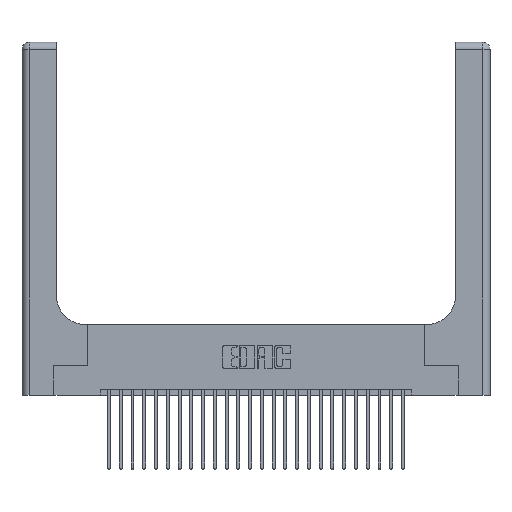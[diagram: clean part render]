
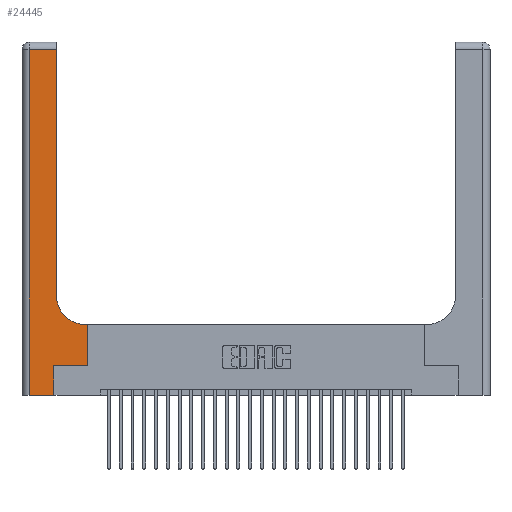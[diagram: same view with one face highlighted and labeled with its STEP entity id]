
A CAD part, top view. The second image highlights one B-rep face of the part: STEP entity #24445.
In plain terms, the highlighted planar face has unit normal (0, 0, 1).
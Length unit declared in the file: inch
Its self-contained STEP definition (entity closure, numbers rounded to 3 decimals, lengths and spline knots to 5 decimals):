
#80 = CARTESIAN_POINT ( 'NONE',  ( 0.06, 2.94, 0.37 ) ) ;
#193 = EDGE_CURVE ( 'NONE', #15924, #9389, #17839, .T. ) ;
#535 = CARTESIAN_POINT ( 'NONE',  ( 0.2915, 3., 0.37 ) ) ;
#788 = DIRECTION ( 'NONE',  ( 0., 1., 0. ) ) ;
#855 = EDGE_CURVE ( 'NONE', #9389, #20515, #4159, .T. ) ;
#867 = CARTESIAN_POINT ( 'NONE',  ( 0., 3., 0.37 ) ) ;
#1269 = VECTOR ( 'NONE', #12294, 39.37008 ) ;
#1270 = ORIENTED_EDGE ( 'NONE', *, *, #2714, .T. ) ;
#1662 = DIRECTION ( 'NONE',  ( 0., 1., 0. ) ) ;
#1924 = CARTESIAN_POINT ( 'NONE',  ( 0.5415, 0.85, 0.37 ) ) ;
#2631 = ORIENTED_EDGE ( 'NONE', *, *, #27684, .T. ) ;
#2714 = EDGE_CURVE ( 'NONE', #18409, #4987, #21042, .T. ) ;
#2763 = VECTOR ( 'NONE', #6389, 39.37008 ) ;
#3029 = ORIENTED_EDGE ( 'NONE', *, *, #6999, .T. ) ;
#3527 = ORIENTED_EDGE ( 'NONE', *, *, #18618, .T. ) ;
#3977 = LINE ( 'NONE', #14565, #25992 ) ;
#4139 = DIRECTION ( 'NONE',  ( 1., 0., 0. ) ) ;
#4159 = LINE ( 'NONE', #6095, #2763 ) ;
#4470 = AXIS2_PLACEMENT_3D ( 'NONE', #867, #7501, #22322 ) ;
#4987 = VERTEX_POINT ( 'NONE', #16318 ) ;
#5152 = CARTESIAN_POINT ( 'NONE',  ( 0., 0., 0.37 ) ) ;
#5237 = LINE ( 'NONE', #7426, #21514 ) ;
#5331 = PLANE ( 'NONE',  #4470 ) ;
#6095 = CARTESIAN_POINT ( 'NONE',  ( 0., 2.94, 0.37 ) ) ;
#6389 = DIRECTION ( 'NONE',  ( -1., 0., 0. ) ) ;
#6818 = EDGE_CURVE ( 'NONE', #16713, #26594, #27409, .T. ) ;
#6999 = EDGE_CURVE ( 'NONE', #4987, #13954, #24064, .T. ) ;
#7273 = AXIS2_PLACEMENT_3D ( 'NONE', #1924, #16900, #4139 ) ;
#7426 = CARTESIAN_POINT ( 'NONE',  ( 0.269, 0., 0.37 ) ) ;
#7501 = DIRECTION ( 'NONE',  ( 0., 0., -1. ) ) ;
#7869 = CARTESIAN_POINT ( 'NONE',  ( 0.2915, 2.94, 0.37 ) ) ;
#9167 = ORIENTED_EDGE ( 'NONE', *, *, #19761, .T. ) ;
#9389 = VERTEX_POINT ( 'NONE', #7869 ) ;
#9625 = ORIENTED_EDGE ( 'NONE', *, *, #6818, .T. ) ;
#10410 = CIRCLE ( 'NONE', #7273, 0.25 ) ;
#10660 = VECTOR ( 'NONE', #19065, 39.37008 ) ;
#11289 = CARTESIAN_POINT ( 'NONE',  ( 0.269, 0., 0.37 ) ) ;
#11667 = VERTEX_POINT ( 'NONE', #24342 ) ;
#11761 = FACE_OUTER_BOUND ( 'NONE', #12996, .T. ) ;
#12276 = ORIENTED_EDGE ( 'NONE', *, *, #855, .T. ) ;
#12294 = DIRECTION ( 'NONE',  ( -1., 0., 0. ) ) ;
#12996 = EDGE_LOOP ( 'NONE', ( #23072, #12276, #9167, #9625, #2631, #3527, #1270, #3029, #24319 ) ) ;
#13675 = CARTESIAN_POINT ( 'NONE',  ( 0.5585, 0.25, 0.37 ) ) ;
#13954 = VERTEX_POINT ( 'NONE', #15726 ) ;
#14565 = CARTESIAN_POINT ( 'NONE',  ( 0.269, 0.25, 0.37 ) ) ;
#14772 = CARTESIAN_POINT ( 'NONE',  ( 0.06, 3., 0.37 ) ) ;
#15379 = VECTOR ( 'NONE', #21538, 39.37008 ) ;
#15726 = CARTESIAN_POINT ( 'NONE',  ( 0.5415, 0.6, 0.37 ) ) ;
#15924 = VERTEX_POINT ( 'NONE', #18438 ) ;
#16037 = VECTOR ( 'NONE', #26257, 39.37008 ) ;
#16318 = CARTESIAN_POINT ( 'NONE',  ( 0.5585, 0.6, 0.37 ) ) ;
#16713 = VERTEX_POINT ( 'NONE', #22496 ) ;
#16900 = DIRECTION ( 'NONE',  ( 0., 0., -1. ) ) ;
#16952 = EDGE_CURVE ( 'NONE', #13954, #15924, #10410, .T. ) ;
#17839 = LINE ( 'NONE', #535, #23477 ) ;
#18409 = VERTEX_POINT ( 'NONE', #13675 ) ;
#18438 = CARTESIAN_POINT ( 'NONE',  ( 0.2915, 0.85, 0.37 ) ) ;
#18618 = EDGE_CURVE ( 'NONE', #11667, #18409, #3977, .T. ) ;
#18850 = DIRECTION ( 'NONE',  ( 1., 0., 0. ) ) ;
#19065 = DIRECTION ( 'NONE',  ( 0., -1., 0. ) ) ;
#19394 = CARTESIAN_POINT ( 'NONE',  ( 0.5585, 0.25, 0.37 ) ) ;
#19761 = EDGE_CURVE ( 'NONE', #20515, #16713, #27603, .T. ) ;
#20515 = VERTEX_POINT ( 'NONE', #80 ) ;
#21042 = LINE ( 'NONE', #19394, #15379 ) ;
#21514 = VECTOR ( 'NONE', #788, 39.37008 ) ;
#21538 = DIRECTION ( 'NONE',  ( 0., 1., 0. ) ) ;
#22322 = DIRECTION ( 'NONE',  ( -1., 0., 0. ) ) ;
#22496 = CARTESIAN_POINT ( 'NONE',  ( 0.06, 0., 0.37 ) ) ;
#22859 = CARTESIAN_POINT ( 'NONE',  ( 0.2915, 0.6, 0.37 ) ) ;
#23072 = ORIENTED_EDGE ( 'NONE', *, *, #193, .T. ) ;
#23477 = VECTOR ( 'NONE', #1662, 39.37008 ) ;
#24064 = LINE ( 'NONE', #22859, #1269 ) ;
#24319 = ORIENTED_EDGE ( 'NONE', *, *, #16952, .T. ) ;
#24342 = CARTESIAN_POINT ( 'NONE',  ( 0.269, 0.25, 0.37 ) ) ;
#24445 = ADVANCED_FACE ( 'NONE', ( #11761 ), #5331, .F. ) ;
#25992 = VECTOR ( 'NONE', #18850, 39.37008 ) ;
#26257 = DIRECTION ( 'NONE',  ( 1., 0., 0. ) ) ;
#26594 = VERTEX_POINT ( 'NONE', #11289 ) ;
#27409 = LINE ( 'NONE', #5152, #16037 ) ;
#27603 = LINE ( 'NONE', #14772, #10660 ) ;
#27684 = EDGE_CURVE ( 'NONE', #26594, #11667, #5237, .T. ) ;
